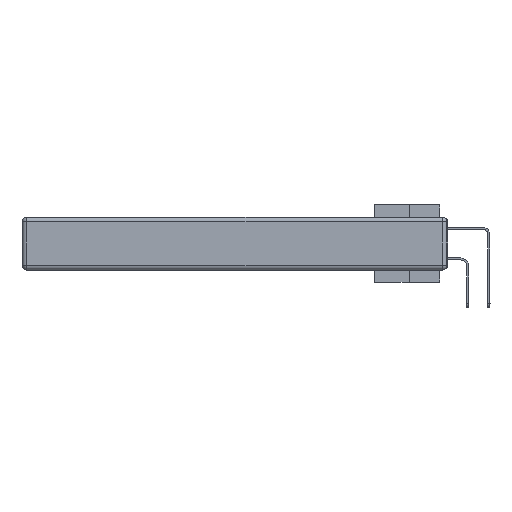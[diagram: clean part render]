
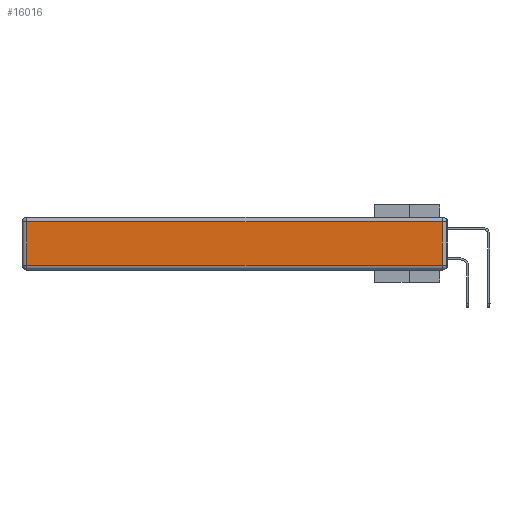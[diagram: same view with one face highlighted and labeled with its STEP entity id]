
A CAD part, left-side view. The second image highlights one B-rep face of the part: STEP entity #16016.
In plain terms, the highlighted planar face has unit normal (-1, 0, 0).
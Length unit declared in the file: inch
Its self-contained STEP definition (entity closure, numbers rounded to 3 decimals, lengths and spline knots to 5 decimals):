
#66 = EDGE_CURVE ( 'NONE', #20480, #18501, #28381, .T. ) ;
#1438 = DIRECTION ( 'NONE',  ( 0., 1., 0. ) ) ;
#1711 = FACE_OUTER_BOUND ( 'NONE', #26131, .T. ) ;
#1780 = CARTESIAN_POINT ( 'NONE',  ( 0., 0.03, -0.343 ) ) ;
#2047 = VECTOR ( 'NONE', #3762, 39.37008 ) ;
#2055 = EDGE_CURVE ( 'NONE', #2480, #20480, #8606, .T. ) ;
#2220 = DIRECTION ( 'NONE',  ( 0., 0., 1. ) ) ;
#2480 = VERTEX_POINT ( 'NONE', #24344 ) ;
#3331 = CARTESIAN_POINT ( 'NONE',  ( 0., 2.72, -0.343 ) ) ;
#3762 = DIRECTION ( 'NONE',  ( 0., -1., 0. ) ) ;
#5088 = VECTOR ( 'NONE', #11094, 39.37008 ) ;
#8606 = LINE ( 'NONE', #24207, #2047 ) ;
#9359 = CARTESIAN_POINT ( 'NONE',  ( 0., 0.03, -0.313 ) ) ;
#11094 = DIRECTION ( 'NONE',  ( 0., 0., -1. ) ) ;
#12545 = DIRECTION ( 'NONE',  ( -1., 0., 0. ) ) ;
#12546 = ORIENTED_EDGE ( 'NONE', *, *, #22395, .T. ) ;
#14257 = CARTESIAN_POINT ( 'NONE',  ( 0., 2.72, -0.03 ) ) ;
#14498 = LINE ( 'NONE', #22384, #22289 ) ;
#15345 = DIRECTION ( 'NONE',  ( 0., 0., 1. ) ) ;
#15450 = CARTESIAN_POINT ( 'NONE',  ( 0., 0., -0.343 ) ) ;
#15534 = VECTOR ( 'NONE', #15345, 39.37008 ) ;
#16016 = ADVANCED_FACE ( 'NONE', ( #1711 ), #28490, .T. ) ;
#16100 = CARTESIAN_POINT ( 'NONE',  ( 0., 0.03, -0.03 ) ) ;
#18501 = VERTEX_POINT ( 'NONE', #16100 ) ;
#19531 = ORIENTED_EDGE ( 'NONE', *, *, #30513, .T. ) ;
#20480 = VERTEX_POINT ( 'NONE', #9359 ) ;
#22289 = VECTOR ( 'NONE', #1438, 39.37008 ) ;
#22384 = CARTESIAN_POINT ( 'NONE',  ( 0., 2.75, -0.03 ) ) ;
#22395 = EDGE_CURVE ( 'NONE', #24771, #2480, #24103, .T. ) ;
#24103 = LINE ( 'NONE', #3331, #5088 ) ;
#24207 = CARTESIAN_POINT ( 'NONE',  ( 0., 0., -0.313 ) ) ;
#24344 = CARTESIAN_POINT ( 'NONE',  ( 0., 2.72, -0.313 ) ) ;
#24771 = VERTEX_POINT ( 'NONE', #14257 ) ;
#26131 = EDGE_LOOP ( 'NONE', ( #29362, #32231, #19531, #12546 ) ) ;
#28381 = LINE ( 'NONE', #1780, #15534 ) ;
#28490 = PLANE ( 'NONE',  #30585 ) ;
#29362 = ORIENTED_EDGE ( 'NONE', *, *, #2055, .T. ) ;
#30513 = EDGE_CURVE ( 'NONE', #18501, #24771, #14498, .T. ) ;
#30585 = AXIS2_PLACEMENT_3D ( 'NONE', #15450, #12545, #2220 ) ;
#32231 = ORIENTED_EDGE ( 'NONE', *, *, #66, .T. ) ;
